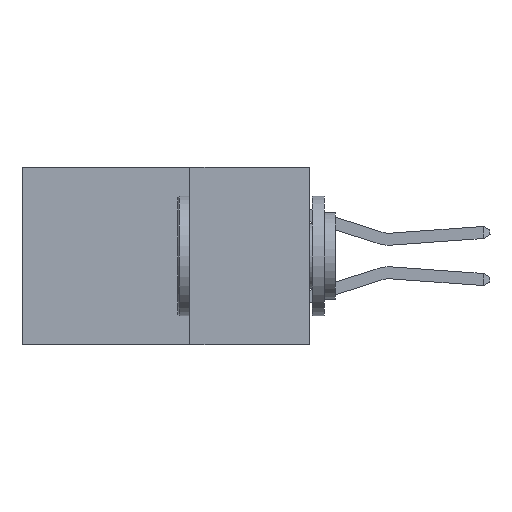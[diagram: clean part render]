
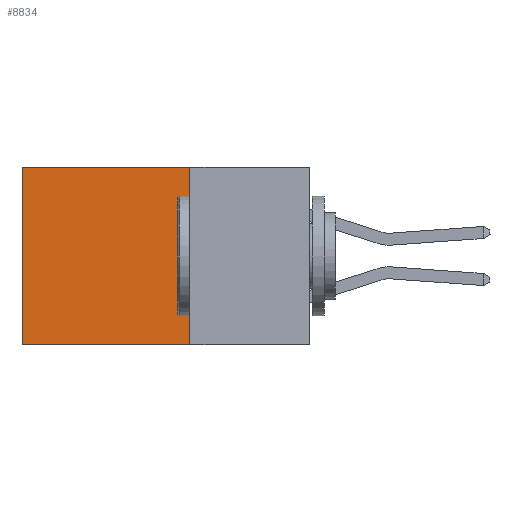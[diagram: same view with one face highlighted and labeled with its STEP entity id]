
A CAD part, left-side view. The second image highlights one B-rep face of the part: STEP entity #8834.
In plain terms, the highlighted planar face has unit normal (-1, 0, 0).
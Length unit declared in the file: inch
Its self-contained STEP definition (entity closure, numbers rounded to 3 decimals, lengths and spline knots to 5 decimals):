
#550 = CARTESIAN_POINT ( 'NONE',  ( 0.2615, 0.6, 0. ) ) ;
#885 = VERTEX_POINT ( 'NONE', #1324 ) ;
#1038 = CARTESIAN_POINT ( 'NONE',  ( 0.2615, 0.25, 0. ) ) ;
#1324 = CARTESIAN_POINT ( 'NONE',  ( 0.2615, 0.25, 0. ) ) ;
#1397 = ORIENTED_EDGE ( 'NONE', *, *, #5478, .F. ) ;
#1501 = LINE ( 'NONE', #8012, #3107 ) ;
#1513 = ORIENTED_EDGE ( 'NONE', *, *, #5315, .T. ) ;
#1563 = CARTESIAN_POINT ( 'NONE',  ( 0.2615, 0.25, -0.37 ) ) ;
#1599 = EDGE_LOOP ( 'NONE', ( #1513, #1397, #6453, #1787 ) ) ;
#1787 = ORIENTED_EDGE ( 'NONE', *, *, #9011, .T. ) ;
#2506 = VERTEX_POINT ( 'NONE', #1563 ) ;
#2508 = DIRECTION ( 'NONE',  ( 0., 1., 0. ) ) ;
#2578 = LINE ( 'NONE', #3407, #2915 ) ;
#2915 = VECTOR ( 'NONE', #9808, 39.37008 ) ;
#3107 = VECTOR ( 'NONE', #10259, 39.37008 ) ;
#3407 = CARTESIAN_POINT ( 'NONE',  ( 0.2615, 0.25, -0.37 ) ) ;
#3709 = PLANE ( 'NONE',  #8309 ) ;
#3831 = DIRECTION ( 'NONE',  ( 0., 0., -1. ) ) ;
#4292 = CARTESIAN_POINT ( 'NONE',  ( 0.2615, 0.6, -0.37 ) ) ;
#4387 = FACE_OUTER_BOUND ( 'NONE', #1599, .T. ) ;
#4621 = CARTESIAN_POINT ( 'NONE',  ( 0.2615, 0.6, -0.37 ) ) ;
#4858 = LINE ( 'NONE', #1038, #5346 ) ;
#4947 = VERTEX_POINT ( 'NONE', #4292 ) ;
#5315 = EDGE_CURVE ( 'NONE', #7961, #4947, #8637, .T. ) ;
#5346 = VECTOR ( 'NONE', #2508, 39.37008 ) ;
#5478 = EDGE_CURVE ( 'NONE', #2506, #4947, #2578, .T. ) ;
#6323 = EDGE_CURVE ( 'NONE', #885, #2506, #1501, .T. ) ;
#6453 = ORIENTED_EDGE ( 'NONE', *, *, #6323, .F. ) ;
#7961 = VERTEX_POINT ( 'NONE', #550 ) ;
#8012 = CARTESIAN_POINT ( 'NONE',  ( 0.2615, 0.25, -0.37 ) ) ;
#8309 = AXIS2_PLACEMENT_3D ( 'NONE', #9130, #9907, #9178 ) ;
#8637 = LINE ( 'NONE', #4621, #9406 ) ;
#8834 = ADVANCED_FACE ( 'NONE', ( #4387 ), #3709, .F. ) ;
#9011 = EDGE_CURVE ( 'NONE', #885, #7961, #4858, .T. ) ;
#9130 = CARTESIAN_POINT ( 'NONE',  ( 0.2615, 0.25, -0.37 ) ) ;
#9178 = DIRECTION ( 'NONE',  ( 0., 0., -1. ) ) ;
#9406 = VECTOR ( 'NONE', #3831, 39.37008 ) ;
#9808 = DIRECTION ( 'NONE',  ( 0., 1., 0. ) ) ;
#9907 = DIRECTION ( 'NONE',  ( 1., 0., 0. ) ) ;
#10259 = DIRECTION ( 'NONE',  ( 0., 0., -1. ) ) ;
